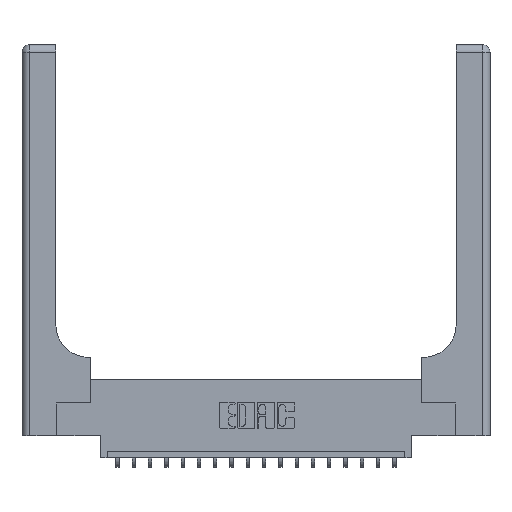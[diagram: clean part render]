
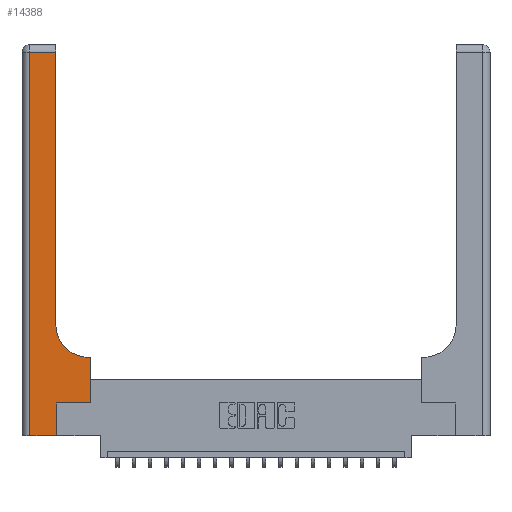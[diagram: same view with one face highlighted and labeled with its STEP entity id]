
A CAD part, top view. The second image highlights one B-rep face of the part: STEP entity #14388.
In plain terms, the highlighted planar face has unit normal (0, 0, 1).
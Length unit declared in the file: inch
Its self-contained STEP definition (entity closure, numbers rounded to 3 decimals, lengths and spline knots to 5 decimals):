
#142 = CARTESIAN_POINT ( 'NONE',  ( 0.265, 0., 0.37 ) ) ;
#811 = ORIENTED_EDGE ( 'NONE', *, *, #7893, .T. ) ;
#884 = ORIENTED_EDGE ( 'NONE', *, *, #19038, .T. ) ;
#1017 = LINE ( 'NONE', #11276, #13988 ) ;
#1129 = VECTOR ( 'NONE', #3597, 39.37008 ) ;
#1449 = DIRECTION ( 'NONE',  ( 1., 0., 0. ) ) ;
#1781 = VERTEX_POINT ( 'NONE', #6230 ) ;
#2109 = EDGE_CURVE ( 'NONE', #1781, #17256, #5123, .T. ) ;
#2543 = DIRECTION ( 'NONE',  ( -1., 0., 0. ) ) ;
#2892 = ORIENTED_EDGE ( 'NONE', *, *, #19551, .T. ) ;
#3150 = ORIENTED_EDGE ( 'NONE', *, *, #7959, .T. ) ;
#3173 = EDGE_LOOP ( 'NONE', ( #3150, #4978, #811, #4745, #884, #2892, #5429, #11879, #4855 ) ) ;
#3488 = CARTESIAN_POINT ( 'NONE',  ( 0.06, 0., 0.37 ) ) ;
#3597 = DIRECTION ( 'NONE',  ( 0., 1., 0. ) ) ;
#3898 = VERTEX_POINT ( 'NONE', #142 ) ;
#4534 = DIRECTION ( 'NONE',  ( 0., -1., 0. ) ) ;
#4745 = ORIENTED_EDGE ( 'NONE', *, *, #13742, .T. ) ;
#4791 = CARTESIAN_POINT ( 'NONE',  ( 0.528, 0.25, 0.37 ) ) ;
#4810 = LINE ( 'NONE', #17301, #13672 ) ;
#4855 = ORIENTED_EDGE ( 'NONE', *, *, #2109, .T. ) ;
#4978 = ORIENTED_EDGE ( 'NONE', *, *, #18694, .T. ) ;
#5123 = CIRCLE ( 'NONE', #10708, 0.25 ) ;
#5414 = CARTESIAN_POINT ( 'NONE',  ( 0.26, 0.85, 0.37 ) ) ;
#5429 = ORIENTED_EDGE ( 'NONE', *, *, #15048, .T. ) ;
#6230 = CARTESIAN_POINT ( 'NONE',  ( 0.51, 0.6, 0.37 ) ) ;
#6360 = LINE ( 'NONE', #20076, #10613 ) ;
#6743 = CARTESIAN_POINT ( 'NONE',  ( 0.528, 0.6, 0.37 ) ) ;
#7118 = LINE ( 'NONE', #8535, #20229 ) ;
#7290 = LINE ( 'NONE', #18261, #9456 ) ;
#7597 = DIRECTION ( 'NONE',  ( 0., 0., -1. ) ) ;
#7893 = EDGE_CURVE ( 'NONE', #11208, #14590, #6360, .T. ) ;
#7959 = EDGE_CURVE ( 'NONE', #17256, #12644, #11253, .T. ) ;
#8025 = AXIS2_PLACEMENT_3D ( 'NONE', #8300, #19476, #14777 ) ;
#8058 = DIRECTION ( 'NONE',  ( 0., 1., 0. ) ) ;
#8158 = VECTOR ( 'NONE', #19092, 39.37008 ) ;
#8300 = CARTESIAN_POINT ( 'NONE',  ( 0., 3., 0.37 ) ) ;
#8302 = DIRECTION ( 'NONE',  ( -1., 0., 0. ) ) ;
#8507 = PLANE ( 'NONE',  #8025 ) ;
#8535 = CARTESIAN_POINT ( 'NONE',  ( 0.265, 0.25, 0.37 ) ) ;
#9456 = VECTOR ( 'NONE', #13435, 39.37008 ) ;
#9752 = VERTEX_POINT ( 'NONE', #6743 ) ;
#9982 = VERTEX_POINT ( 'NONE', #4791 ) ;
#10613 = VECTOR ( 'NONE', #4534, 39.37008 ) ;
#10700 = CARTESIAN_POINT ( 'NONE',  ( 0.06, 2.94, 0.37 ) ) ;
#10708 = AXIS2_PLACEMENT_3D ( 'NONE', #11831, #7597, #1449 ) ;
#11074 = EDGE_CURVE ( 'NONE', #9752, #1781, #15233, .T. ) ;
#11208 = VERTEX_POINT ( 'NONE', #10700 ) ;
#11253 = LINE ( 'NONE', #19261, #1129 ) ;
#11276 = CARTESIAN_POINT ( 'NONE',  ( 0., 2.94, 0.37 ) ) ;
#11338 = CARTESIAN_POINT ( 'NONE',  ( 0.265, 0.25, 0.37 ) ) ;
#11383 = VECTOR ( 'NONE', #2543, 39.37008 ) ;
#11416 = DIRECTION ( 'NONE',  ( 1., 0., 0. ) ) ;
#11482 = FACE_OUTER_BOUND ( 'NONE', #3173, .T. ) ;
#11831 = CARTESIAN_POINT ( 'NONE',  ( 0.51, 0.85, 0.37 ) ) ;
#11879 = ORIENTED_EDGE ( 'NONE', *, *, #11074, .T. ) ;
#12644 = VERTEX_POINT ( 'NONE', #17971 ) ;
#12837 = CARTESIAN_POINT ( 'NONE',  ( 0., 0., 0.37 ) ) ;
#13435 = DIRECTION ( 'NONE',  ( 0., 1., 0. ) ) ;
#13672 = VECTOR ( 'NONE', #8058, 39.37008 ) ;
#13742 = EDGE_CURVE ( 'NONE', #14590, #3898, #15943, .T. ) ;
#13988 = VECTOR ( 'NONE', #8302, 39.37008 ) ;
#14388 = ADVANCED_FACE ( 'NONE', ( #11482 ), #8507, .F. ) ;
#14590 = VERTEX_POINT ( 'NONE', #3488 ) ;
#14777 = DIRECTION ( 'NONE',  ( -1., 0., 0. ) ) ;
#15048 = EDGE_CURVE ( 'NONE', #9982, #9752, #7290, .T. ) ;
#15233 = LINE ( 'NONE', #19839, #11383 ) ;
#15943 = LINE ( 'NONE', #12837, #8158 ) ;
#17017 = VERTEX_POINT ( 'NONE', #11338 ) ;
#17256 = VERTEX_POINT ( 'NONE', #5414 ) ;
#17301 = CARTESIAN_POINT ( 'NONE',  ( 0.265, 0., 0.37 ) ) ;
#17971 = CARTESIAN_POINT ( 'NONE',  ( 0.26, 2.94, 0.37 ) ) ;
#18261 = CARTESIAN_POINT ( 'NONE',  ( 0.528, 0.25, 0.37 ) ) ;
#18694 = EDGE_CURVE ( 'NONE', #12644, #11208, #1017, .T. ) ;
#19038 = EDGE_CURVE ( 'NONE', #3898, #17017, #4810, .T. ) ;
#19092 = DIRECTION ( 'NONE',  ( 1., 0., 0. ) ) ;
#19261 = CARTESIAN_POINT ( 'NONE',  ( 0.26, 3., 0.37 ) ) ;
#19476 = DIRECTION ( 'NONE',  ( 0., 0., -1. ) ) ;
#19551 = EDGE_CURVE ( 'NONE', #17017, #9982, #7118, .T. ) ;
#19839 = CARTESIAN_POINT ( 'NONE',  ( 0.26, 0.6, 0.37 ) ) ;
#20076 = CARTESIAN_POINT ( 'NONE',  ( 0.06, 3., 0.37 ) ) ;
#20229 = VECTOR ( 'NONE', #11416, 39.37008 ) ;
